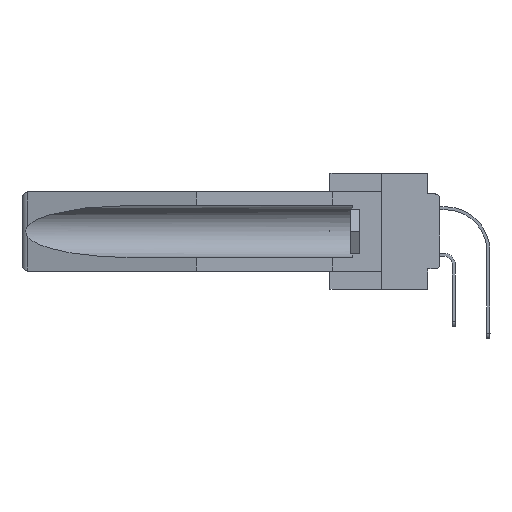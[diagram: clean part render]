
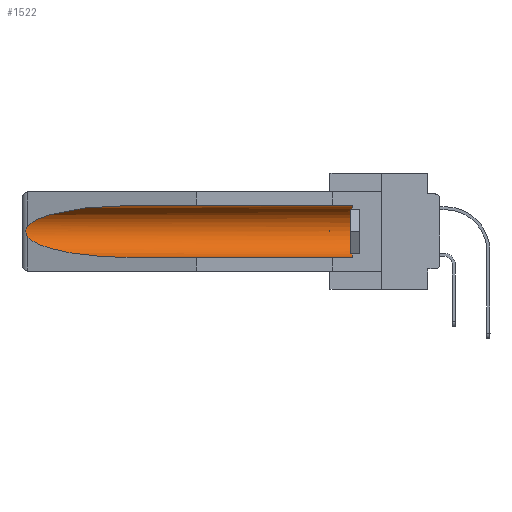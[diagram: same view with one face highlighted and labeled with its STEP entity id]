
A CAD part, left-side view. The second image highlights one B-rep face of the part: STEP entity #1522.
In plain terms, the highlighted cylindrical face has radius 2.857 mm (diameter 5.715 mm), a partial arc.
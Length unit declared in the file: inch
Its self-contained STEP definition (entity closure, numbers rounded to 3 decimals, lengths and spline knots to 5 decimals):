
#493 = CARTESIAN_POINT ( 'NONE',  ( 0.2673, 1.5327, -0.16383 ) ) ;
#1449 = VECTOR ( 'NONE', #5464, 39.37008 ) ;
#1522 = ADVANCED_FACE ( 'NONE', ( #24860 ), #37611, .F. ) ;
#3325 = CARTESIAN_POINT ( 'NONE',  ( 0.26537, 1.52718, -0.19328 ) ) ;
#3365 = VERTEX_POINT ( 'NONE', #15920 ) ;
#4027 = VECTOR ( 'NONE', #31813, 39.37008 ) ;
#4230 = CARTESIAN_POINT ( 'NONE',  ( 0.2673, 1.53269, -0.17917 ) ) ;
#5464 = DIRECTION ( 'NONE',  ( 0., 1., 0. ) ) ;
#6137 = EDGE_CURVE ( 'NONE', #25489, #3365, #28663, .T. ) ;
#6673 = CARTESIAN_POINT ( 'NONE',  ( 0.155, 0.126, -0.284 ) ) ;
#7203 = EDGE_CURVE ( 'NONE', #25489, #9591, #28886, .T. ) ;
#8328 = ORIENTED_EDGE ( 'NONE', *, *, #7203, .F. ) ;
#9591 = VERTEX_POINT ( 'NONE', #15559 ) ;
#9985 = EDGE_CURVE ( 'NONE', #3365, #10985, #37013, .T. ) ;
#10764 = EDGE_LOOP ( 'NONE', ( #19126, #34842, #30314, #8328, #24489, #31213 ) ) ;
#10985 = VERTEX_POINT ( 'NONE', #28816 ) ;
#13206 = CARTESIAN_POINT ( 'NONE',  ( 0.2675, 1.53308, -0.17534 ) ) ;
#15436 = DIRECTION ( 'NONE',  ( 0., 0., 1. ) ) ;
#15559 = CARTESIAN_POINT ( 'NONE',  ( 0.155, 1.07973, -0.284 ) ) ;
#15920 = CARTESIAN_POINT ( 'NONE',  ( 0.155, 0.126, -0.059 ) ) ;
#16045 = CARTESIAN_POINT ( 'NONE',  ( 0.21114, 1.30732, -0.284 ) ) ;
#16119 = CARTESIAN_POINT ( 'NONE',  ( 0.155, -0.30754, -0.284 ) ) ;
#16337 = CARTESIAN_POINT ( 'NONE',  ( 0.26597, 1.52961, -0.15275 ) ) ;
#16539 = CARTESIAN_POINT ( 'NONE',  ( 0.26537, 1.52718, -0.14972 ) ) ;
#16944 = CARTESIAN_POINT ( 'NONE',  ( 0.26597, 1.5296, -0.19026 ) ) ;
#17501 = B_SPLINE_CURVE_WITH_KNOTS ( 'NONE', 3,
 ( #16539, #16337, #32851, #493, #26371, #13206, #4230, #25968, #16944, #39304 ),
 .UNSPECIFIED., .F., .F.,
 ( 4, 2, 2, 2, 4 ),
 ( 0., 0.00029, 0.00058, 0.00087, 0.00117 ),
 .UNSPECIFIED. ) ;
#19003 =( BOUNDED_CURVE ( )  B_SPLINE_CURVE ( 3, ( #19474, #35364, #26378, #39114 ),
 .UNSPECIFIED., .F., .F. ) 
 B_SPLINE_CURVE_WITH_KNOTS ( ( 4, 4 ),
 ( 4.71239, 6.08839 ),
 .UNSPECIFIED. ) 
 CURVE ( )  GEOMETRIC_REPRESENTATION_ITEM ( )  RATIONAL_B_SPLINE_CURVE ( ( 1., 0.848, 0.848, 1. ) ) 
 REPRESENTATION_ITEM ( '' )  );
#19126 = ORIENTED_EDGE ( 'NONE', *, *, #28460, .T. ) ;
#19474 = CARTESIAN_POINT ( 'NONE',  ( 0.155, 1.07973, -0.059 ) ) ;
#19931 = CARTESIAN_POINT ( 'NONE',  ( 0.155, 0.126, -0.1715 ) ) ;
#20138 = DIRECTION ( 'NONE',  ( 0., 0., 1. ) ) ;
#20638 = CARTESIAN_POINT ( 'NONE',  ( 0.26537, 1.52718, -0.19328 ) ) ;
#21120 = CARTESIAN_POINT ( 'NONE',  ( 0.155, -0.30754, -0.059 ) ) ;
#21709 = CARTESIAN_POINT ( 'NONE',  ( 0.155, -0.30754, -0.1715 ) ) ;
#24489 = ORIENTED_EDGE ( 'NONE', *, *, #6137, .T. ) ;
#24849 = CARTESIAN_POINT ( 'NONE',  ( 0.155, 1.07973, -0.284 ) ) ;
#24860 = FACE_OUTER_BOUND ( 'NONE', #10764, .T. ) ;
#25213 = AXIS2_PLACEMENT_3D ( 'NONE', #21709, #34472, #15436 ) ;
#25489 = VERTEX_POINT ( 'NONE', #6673 ) ;
#25599 = VERTEX_POINT ( 'NONE', #20638 ) ;
#25968 = CARTESIAN_POINT ( 'NONE',  ( 0.26655, 1.53094, -0.18657 ) ) ;
#26371 = CARTESIAN_POINT ( 'NONE',  ( 0.2675, 1.53308, -0.16763 ) ) ;
#26378 = CARTESIAN_POINT ( 'NONE',  ( 0.25451, 1.48313, -0.09465 ) ) ;
#26849 = VERTEX_POINT ( 'NONE', #39110 ) ;
#26893 = EDGE_CURVE ( 'NONE', #26849, #25599, #17501, .T. ) ;
#28460 = EDGE_CURVE ( 'NONE', #10985, #26849, #19003, .T. ) ;
#28663 = CIRCLE ( 'NONE', #39993, 0.1125 ) ;
#28816 = CARTESIAN_POINT ( 'NONE',  ( 0.155, 1.07973, -0.059 ) ) ;
#28886 = LINE ( 'NONE', #16119, #4027 ) ;
#30197 = DIRECTION ( 'NONE',  ( 0., -1., 0. ) ) ;
#30314 = ORIENTED_EDGE ( 'NONE', *, *, #33502, .T. ) ;
#31213 = ORIENTED_EDGE ( 'NONE', *, *, #9985, .T. ) ;
#31813 = DIRECTION ( 'NONE',  ( 0., 1., 0. ) ) ;
#32851 = CARTESIAN_POINT ( 'NONE',  ( 0.26654, 1.53092, -0.15636 ) ) ;
#33502 = EDGE_CURVE ( 'NONE', #25599, #9591, #36094, .T. ) ;
#34472 = DIRECTION ( 'NONE',  ( 0., 1., 0. ) ) ;
#34842 = ORIENTED_EDGE ( 'NONE', *, *, #26893, .T. ) ;
#35364 = CARTESIAN_POINT ( 'NONE',  ( 0.21114, 1.30732, -0.059 ) ) ;
#36094 =( BOUNDED_CURVE ( )  B_SPLINE_CURVE ( 3, ( #3325, #37599, #16045, #24849 ),
 .UNSPECIFIED., .F., .F. ) 
 B_SPLINE_CURVE_WITH_KNOTS ( ( 4, 4 ),
 ( 0.1948, 1.5708 ),
 .UNSPECIFIED. ) 
 CURVE ( )  GEOMETRIC_REPRESENTATION_ITEM ( )  RATIONAL_B_SPLINE_CURVE ( ( 1., 0.848, 0.848, 1. ) ) 
 REPRESENTATION_ITEM ( '' )  );
#37013 = LINE ( 'NONE', #21120, #1449 ) ;
#37599 = CARTESIAN_POINT ( 'NONE',  ( 0.25451, 1.48313, -0.24835 ) ) ;
#37611 = CYLINDRICAL_SURFACE ( 'NONE', #25213, 0.1125 ) ;
#39110 = CARTESIAN_POINT ( 'NONE',  ( 0.26537, 1.52718, -0.14972 ) ) ;
#39114 = CARTESIAN_POINT ( 'NONE',  ( 0.26537, 1.52718, -0.14972 ) ) ;
#39304 = CARTESIAN_POINT ( 'NONE',  ( 0.26537, 1.52718, -0.19328 ) ) ;
#39993 = AXIS2_PLACEMENT_3D ( 'NONE', #19931, #30197, #20138 ) ;
